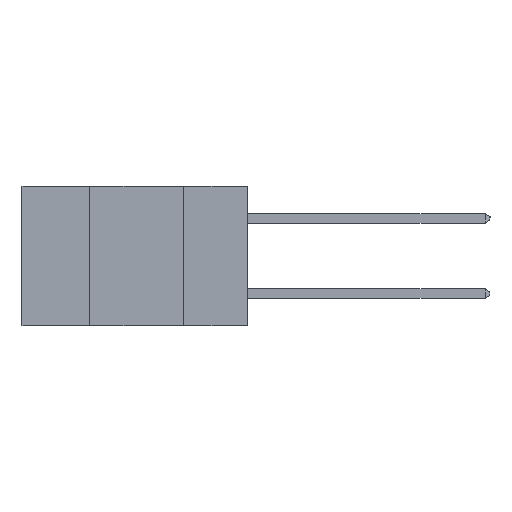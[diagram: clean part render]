
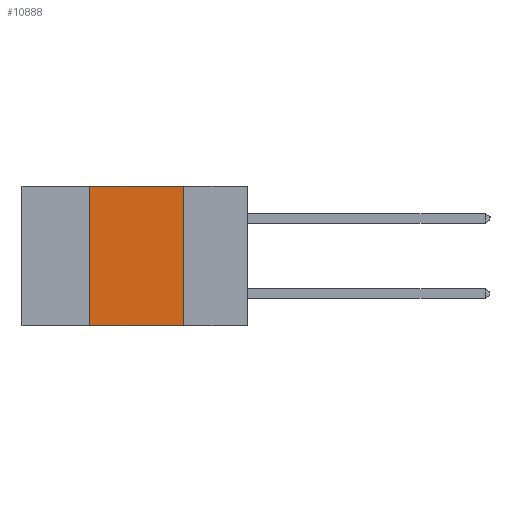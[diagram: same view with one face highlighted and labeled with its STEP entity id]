
A CAD part, left-side view. The second image highlights one B-rep face of the part: STEP entity #10888.
In plain terms, the highlighted planar face has unit normal (-1, 0, 0).
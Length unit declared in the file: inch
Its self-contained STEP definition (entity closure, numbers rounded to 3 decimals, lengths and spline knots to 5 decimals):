
#619 = ORIENTED_EDGE ( 'NONE', *, *, #13205, .F. ) ;
#1682 = EDGE_CURVE ( 'NONE', #6544, #16470, #4893, .T. ) ;
#2439 = DIRECTION ( 'NONE',  ( 0., 0., -1. ) ) ;
#2536 = DIRECTION ( 'NONE',  ( 1., 0., 0. ) ) ;
#2932 = EDGE_LOOP ( 'NONE', ( #619, #9126, #5985, #9187 ) ) ;
#3343 = CARTESIAN_POINT ( 'NONE',  ( 0., 0.42, 0. ) ) ;
#3844 = DIRECTION ( 'NONE',  ( 0., -1., 0. ) ) ;
#4413 = VECTOR ( 'NONE', #11432, 39.37008 ) ;
#4893 = LINE ( 'NONE', #14701, #4413 ) ;
#5345 = DIRECTION ( 'NONE',  ( 0., 0., 1. ) ) ;
#5677 = LINE ( 'NONE', #16906, #20441 ) ;
#5693 = CARTESIAN_POINT ( 'NONE',  ( 0., 0.6, 0. ) ) ;
#5985 = ORIENTED_EDGE ( 'NONE', *, *, #15079, .F. ) ;
#6495 = EDGE_CURVE ( 'NONE', #6871, #6687, #5677, .T. ) ;
#6544 = VERTEX_POINT ( 'NONE', #8504 ) ;
#6687 = VERTEX_POINT ( 'NONE', #16697 ) ;
#6871 = VERTEX_POINT ( 'NONE', #3343 ) ;
#8269 = VECTOR ( 'NONE', #5345, 39.37008 ) ;
#8504 = CARTESIAN_POINT ( 'NONE',  ( 0., 0.42, -0.37 ) ) ;
#9126 = ORIENTED_EDGE ( 'NONE', *, *, #6495, .F. ) ;
#9187 = ORIENTED_EDGE ( 'NONE', *, *, #1682, .T. ) ;
#9264 = VECTOR ( 'NONE', #10261, 39.37008 ) ;
#9405 = FACE_OUTER_BOUND ( 'NONE', #2932, .T. ) ;
#10261 = DIRECTION ( 'NONE',  ( 0., 0., -1. ) ) ;
#10888 = ADVANCED_FACE ( 'NONE', ( #9405 ), #20651, .F. ) ;
#11432 = DIRECTION ( 'NONE',  ( 0., -1., 0. ) ) ;
#13205 = EDGE_CURVE ( 'NONE', #6687, #16470, #18250, .T. ) ;
#13554 = CARTESIAN_POINT ( 'NONE',  ( 0., 0.17, -0.37 ) ) ;
#14701 = CARTESIAN_POINT ( 'NONE',  ( 0., 0.6, -0.37 ) ) ;
#15079 = EDGE_CURVE ( 'NONE', #6544, #6871, #18553, .T. ) ;
#15283 = CARTESIAN_POINT ( 'NONE',  ( 0., 0.42, -0.37 ) ) ;
#15988 = CARTESIAN_POINT ( 'NONE',  ( 0., 0.17, -0.37 ) ) ;
#16470 = VERTEX_POINT ( 'NONE', #15988 ) ;
#16697 = CARTESIAN_POINT ( 'NONE',  ( 0., 0.17, 0. ) ) ;
#16906 = CARTESIAN_POINT ( 'NONE',  ( 0., 0.6, 0. ) ) ;
#18250 = LINE ( 'NONE', #13554, #9264 ) ;
#18553 = LINE ( 'NONE', #15283, #8269 ) ;
#18973 = AXIS2_PLACEMENT_3D ( 'NONE', #5693, #2536, #2439 ) ;
#20441 = VECTOR ( 'NONE', #3844, 39.37008 ) ;
#20651 = PLANE ( 'NONE',  #18973 ) ;
